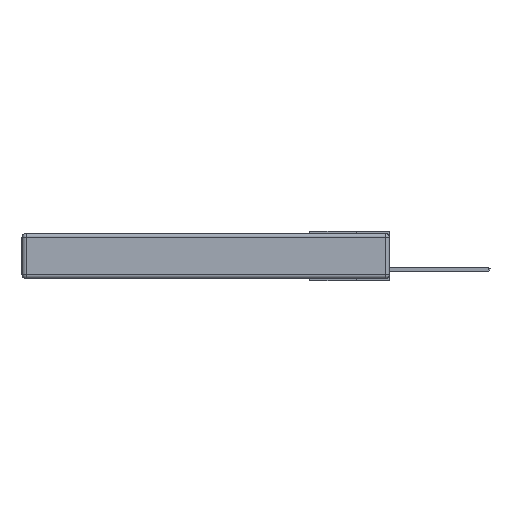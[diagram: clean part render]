
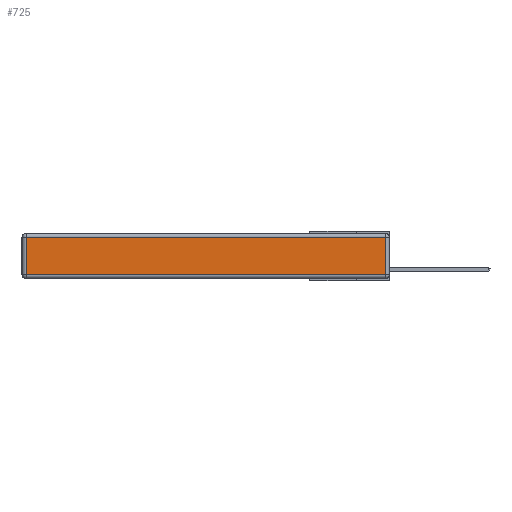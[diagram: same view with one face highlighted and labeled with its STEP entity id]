
A CAD part, left-side view. The second image highlights one B-rep face of the part: STEP entity #725.
In plain terms, the highlighted planar face has unit normal (-1, 0, 0).
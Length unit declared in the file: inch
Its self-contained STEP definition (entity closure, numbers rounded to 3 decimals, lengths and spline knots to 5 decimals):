
#52 = LINE ( 'NONE', #18202, #13365 ) ;
#510 = VECTOR ( 'NONE', #3562, 39.37008 ) ;
#725 = ADVANCED_FACE ( 'NONE', ( #14938 ), #14333, .T. ) ;
#2916 = ORIENTED_EDGE ( 'NONE', *, *, #16313, .T. ) ;
#3562 = DIRECTION ( 'NONE',  ( 0., 0., -1. ) ) ;
#4034 = VERTEX_POINT ( 'NONE', #7995 ) ;
#4066 = LINE ( 'NONE', #5627, #14993 ) ;
#5627 = CARTESIAN_POINT ( 'NONE',  ( 0., 2.75, -0.03 ) ) ;
#5872 = AXIS2_PLACEMENT_3D ( 'NONE', #8211, #12810, #18837 ) ;
#6625 = EDGE_CURVE ( 'NONE', #4034, #13188, #4066, .T. ) ;
#6871 = ORIENTED_EDGE ( 'NONE', *, *, #9098, .T. ) ;
#6966 = VERTEX_POINT ( 'NONE', #9220 ) ;
#7676 = ORIENTED_EDGE ( 'NONE', *, *, #10034, .T. ) ;
#7995 = CARTESIAN_POINT ( 'NONE',  ( 0., 0.03, -0.03 ) ) ;
#8211 = CARTESIAN_POINT ( 'NONE',  ( 0., 0., -0.343 ) ) ;
#8245 = CARTESIAN_POINT ( 'NONE',  ( 0., 0.03, -0.313 ) ) ;
#8757 = CARTESIAN_POINT ( 'NONE',  ( 0., 2.72, -0.03 ) ) ;
#9098 = EDGE_CURVE ( 'NONE', #14747, #4034, #52, .T. ) ;
#9220 = CARTESIAN_POINT ( 'NONE',  ( 0., 2.72, -0.313 ) ) ;
#9269 = DIRECTION ( 'NONE',  ( 0., -1., 0. ) ) ;
#9618 = ORIENTED_EDGE ( 'NONE', *, *, #6625, .T. ) ;
#9762 = VECTOR ( 'NONE', #9269, 39.37008 ) ;
#10034 = EDGE_CURVE ( 'NONE', #13188, #6966, #17809, .T. ) ;
#12810 = DIRECTION ( 'NONE',  ( -1., 0., 0. ) ) ;
#13188 = VERTEX_POINT ( 'NONE', #8757 ) ;
#13365 = VECTOR ( 'NONE', #19570, 39.37008 ) ;
#13851 = CARTESIAN_POINT ( 'NONE',  ( 0., 0., -0.313 ) ) ;
#14333 = PLANE ( 'NONE',  #5872 ) ;
#14747 = VERTEX_POINT ( 'NONE', #8245 ) ;
#14938 = FACE_OUTER_BOUND ( 'NONE', #18102, .T. ) ;
#14993 = VECTOR ( 'NONE', #19083, 39.37008 ) ;
#15598 = CARTESIAN_POINT ( 'NONE',  ( 0., 2.72, -0.343 ) ) ;
#16313 = EDGE_CURVE ( 'NONE', #6966, #14747, #17620, .T. ) ;
#17620 = LINE ( 'NONE', #13851, #9762 ) ;
#17809 = LINE ( 'NONE', #15598, #510 ) ;
#18102 = EDGE_LOOP ( 'NONE', ( #2916, #6871, #9618, #7676 ) ) ;
#18202 = CARTESIAN_POINT ( 'NONE',  ( 0., 0.03, -0.343 ) ) ;
#18837 = DIRECTION ( 'NONE',  ( 0., 0., 1. ) ) ;
#19083 = DIRECTION ( 'NONE',  ( 0., 1., 0. ) ) ;
#19570 = DIRECTION ( 'NONE',  ( 0., 0., 1. ) ) ;
